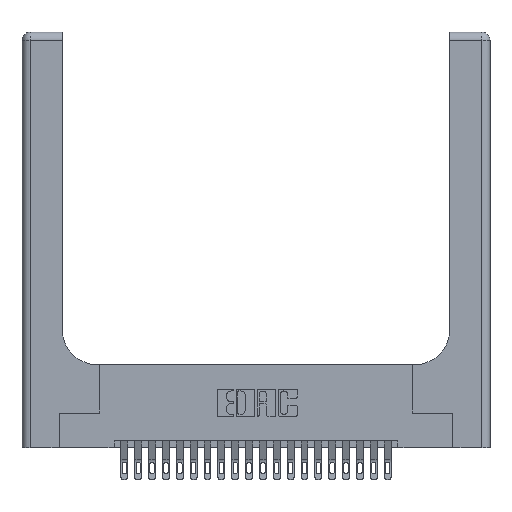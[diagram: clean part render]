
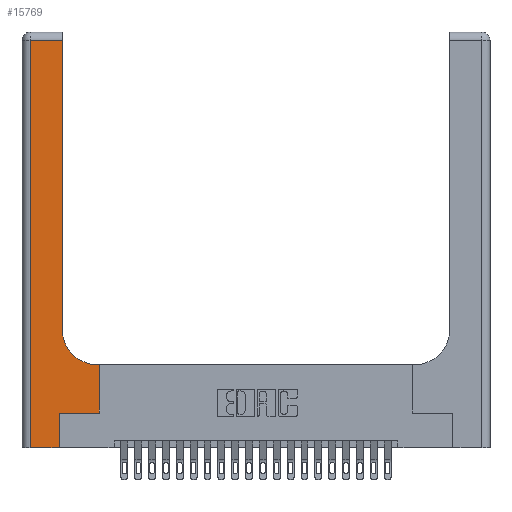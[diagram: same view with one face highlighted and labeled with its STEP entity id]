
A CAD part, top view. The second image highlights one B-rep face of the part: STEP entity #15769.
In plain terms, the highlighted planar face has unit normal (0, 0, 1).
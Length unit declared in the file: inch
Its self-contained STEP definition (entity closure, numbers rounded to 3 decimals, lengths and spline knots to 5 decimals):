
#357 = EDGE_CURVE ( 'NONE', #4583, #14884, #23772, .T. ) ;
#372 = LINE ( 'NONE', #1743, #24039 ) ;
#951 = EDGE_CURVE ( 'NONE', #1400, #4583, #12034, .T. ) ;
#1400 = VERTEX_POINT ( 'NONE', #21146 ) ;
#1426 = DIRECTION ( 'NONE',  ( -1., 0., 0. ) ) ;
#1743 = CARTESIAN_POINT ( 'NONE',  ( 0.2915, 0.6, 0.37 ) ) ;
#1776 = CARTESIAN_POINT ( 'NONE',  ( 0.5415, 0.6, 0.37 ) ) ;
#1943 = EDGE_CURVE ( 'NONE', #4286, #24036, #5256, .T. ) ;
#2433 = CARTESIAN_POINT ( 'NONE',  ( 0., 0., 0.37 ) ) ;
#2462 = ORIENTED_EDGE ( 'NONE', *, *, #1943, .T. ) ;
#3068 = DIRECTION ( 'NONE',  ( 0., 0., -1. ) ) ;
#4136 = AXIS2_PLACEMENT_3D ( 'NONE', #14232, #3068, #16123 ) ;
#4263 = CARTESIAN_POINT ( 'NONE',  ( 0.2915, 0.85, 0.37 ) ) ;
#4286 = VERTEX_POINT ( 'NONE', #22082 ) ;
#4583 = VERTEX_POINT ( 'NONE', #13796 ) ;
#4852 = CARTESIAN_POINT ( 'NONE',  ( 0.269, 0., 0.37 ) ) ;
#5198 = CARTESIAN_POINT ( 'NONE',  ( 0.269, 0., 0.37 ) ) ;
#5256 = LINE ( 'NONE', #2433, #19575 ) ;
#5786 = CARTESIAN_POINT ( 'NONE',  ( 0.5585, 0.6, 0.37 ) ) ;
#5834 = ORIENTED_EDGE ( 'NONE', *, *, #8201, .T. ) ;
#5950 = LINE ( 'NONE', #4852, #10318 ) ;
#6746 = VECTOR ( 'NONE', #18706, 39.37008 ) ;
#7255 = EDGE_CURVE ( 'NONE', #20150, #4286, #13436, .T. ) ;
#7525 = VERTEX_POINT ( 'NONE', #17934 ) ;
#7603 = ORIENTED_EDGE ( 'NONE', *, *, #12549, .T. ) ;
#7605 = DIRECTION ( 'NONE',  ( 1., 0., 0. ) ) ;
#7731 = CARTESIAN_POINT ( 'NONE',  ( 0.269, 0.25, 0.37 ) ) ;
#7792 = PLANE ( 'NONE',  #22249 ) ;
#7899 = ORIENTED_EDGE ( 'NONE', *, *, #7255, .T. ) ;
#8201 = EDGE_CURVE ( 'NONE', #22896, #21738, #13395, .T. ) ;
#9197 = ORIENTED_EDGE ( 'NONE', *, *, #357, .T. ) ;
#9388 = CARTESIAN_POINT ( 'NONE',  ( 0.2915, 3., 0.37 ) ) ;
#9660 = DIRECTION ( 'NONE',  ( -1., 0., 0. ) ) ;
#10318 = VECTOR ( 'NONE', #16051, 39.37008 ) ;
#10549 = ORIENTED_EDGE ( 'NONE', *, *, #21672, .T. ) ;
#10700 = CARTESIAN_POINT ( 'NONE',  ( 0., 2.94, 0.37 ) ) ;
#10958 = ORIENTED_EDGE ( 'NONE', *, *, #951, .T. ) ;
#12034 = LINE ( 'NONE', #7731, #12629 ) ;
#12326 = LINE ( 'NONE', #9388, #6746 ) ;
#12509 = ORIENTED_EDGE ( 'NONE', *, *, #16006, .T. ) ;
#12549 = EDGE_CURVE ( 'NONE', #7525, #20150, #23466, .T. ) ;
#12629 = VECTOR ( 'NONE', #7605, 39.37008 ) ;
#12867 = VECTOR ( 'NONE', #22633, 39.37008 ) ;
#12923 = DIRECTION ( 'NONE',  ( -1., 0., 0. ) ) ;
#12946 = VECTOR ( 'NONE', #1426, 39.37008 ) ;
#13056 = EDGE_CURVE ( 'NONE', #21738, #7525, #12326, .T. ) ;
#13059 = EDGE_LOOP ( 'NONE', ( #14958, #7603, #7899, #2462, #12509, #10958, #9197, #10549, #5834 ) ) ;
#13395 = CIRCLE ( 'NONE', #4136, 0.25 ) ;
#13436 = LINE ( 'NONE', #17064, #12867 ) ;
#13796 = CARTESIAN_POINT ( 'NONE',  ( 0.5585, 0.25, 0.37 ) ) ;
#13809 = VECTOR ( 'NONE', #16418, 39.37008 ) ;
#14232 = CARTESIAN_POINT ( 'NONE',  ( 0.5415, 0.85, 0.37 ) ) ;
#14884 = VERTEX_POINT ( 'NONE', #5786 ) ;
#14958 = ORIENTED_EDGE ( 'NONE', *, *, #13056, .T. ) ;
#15029 = FACE_OUTER_BOUND ( 'NONE', #13059, .T. ) ;
#15769 = ADVANCED_FACE ( 'NONE', ( #15029 ), #7792, .F. ) ;
#16006 = EDGE_CURVE ( 'NONE', #24036, #1400, #5950, .T. ) ;
#16051 = DIRECTION ( 'NONE',  ( 0., 1., 0. ) ) ;
#16123 = DIRECTION ( 'NONE',  ( 1., 0., 0. ) ) ;
#16389 = CARTESIAN_POINT ( 'NONE',  ( 0.5585, 0.25, 0.37 ) ) ;
#16418 = DIRECTION ( 'NONE',  ( 0., 1., 0. ) ) ;
#16972 = CARTESIAN_POINT ( 'NONE',  ( 0., 3., 0.37 ) ) ;
#17064 = CARTESIAN_POINT ( 'NONE',  ( 0.06, 3., 0.37 ) ) ;
#17934 = CARTESIAN_POINT ( 'NONE',  ( 0.2915, 2.94, 0.37 ) ) ;
#18706 = DIRECTION ( 'NONE',  ( 0., 1., 0. ) ) ;
#19575 = VECTOR ( 'NONE', #23031, 39.37008 ) ;
#20150 = VERTEX_POINT ( 'NONE', #20822 ) ;
#20822 = CARTESIAN_POINT ( 'NONE',  ( 0.06, 2.94, 0.37 ) ) ;
#20884 = DIRECTION ( 'NONE',  ( 0., 0., -1. ) ) ;
#21146 = CARTESIAN_POINT ( 'NONE',  ( 0.269, 0.25, 0.37 ) ) ;
#21672 = EDGE_CURVE ( 'NONE', #14884, #22896, #372, .T. ) ;
#21738 = VERTEX_POINT ( 'NONE', #4263 ) ;
#22082 = CARTESIAN_POINT ( 'NONE',  ( 0.06, 0., 0.37 ) ) ;
#22249 = AXIS2_PLACEMENT_3D ( 'NONE', #16972, #20884, #9660 ) ;
#22633 = DIRECTION ( 'NONE',  ( 0., -1., 0. ) ) ;
#22896 = VERTEX_POINT ( 'NONE', #1776 ) ;
#23031 = DIRECTION ( 'NONE',  ( 1., 0., 0. ) ) ;
#23466 = LINE ( 'NONE', #10700, #12946 ) ;
#23772 = LINE ( 'NONE', #16389, #13809 ) ;
#24036 = VERTEX_POINT ( 'NONE', #5198 ) ;
#24039 = VECTOR ( 'NONE', #12923, 39.37008 ) ;
